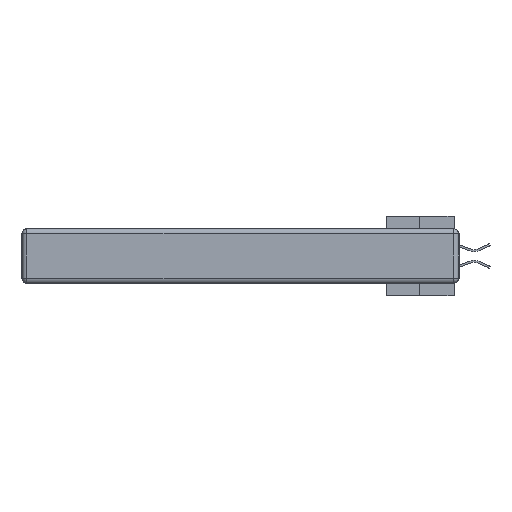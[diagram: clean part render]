
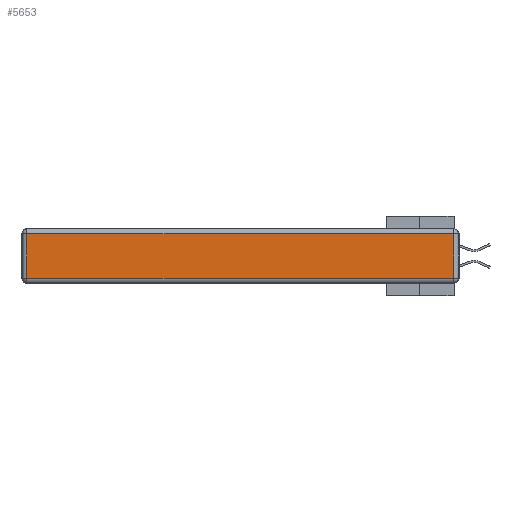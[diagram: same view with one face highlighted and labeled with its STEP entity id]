
A CAD part, left-side view. The second image highlights one B-rep face of the part: STEP entity #5653.
In plain terms, the highlighted planar face has unit normal (-1, 0, 0).
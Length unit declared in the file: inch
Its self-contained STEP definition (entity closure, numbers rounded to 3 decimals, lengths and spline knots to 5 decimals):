
#167 = VECTOR ( 'NONE', #23515, 39.37008 ) ;
#556 = VERTEX_POINT ( 'NONE', #31335 ) ;
#727 = EDGE_LOOP ( 'NONE', ( #11706, #19733, #2817, #20177 ) ) ;
#2817 = ORIENTED_EDGE ( 'NONE', *, *, #37532, .T. ) ;
#2846 = LINE ( 'NONE', #37188, #167 ) ;
#2944 = EDGE_CURVE ( 'NONE', #8887, #556, #6244, .T. ) ;
#5043 = VERTEX_POINT ( 'NONE', #32799 ) ;
#5653 = ADVANCED_FACE ( 'NONE', ( #38411 ), #18246, .T. ) ;
#5727 = CARTESIAN_POINT ( 'NONE',  ( 0., 0.03, -0.343 ) ) ;
#6244 = LINE ( 'NONE', #14846, #38567 ) ;
#8887 = VERTEX_POINT ( 'NONE', #13700 ) ;
#9393 = EDGE_CURVE ( 'NONE', #29796, #8887, #13921, .T. ) ;
#11181 = AXIS2_PLACEMENT_3D ( 'NONE', #21705, #21859, #15105 ) ;
#11333 = DIRECTION ( 'NONE',  ( 0., -1., 0. ) ) ;
#11706 = ORIENTED_EDGE ( 'NONE', *, *, #2944, .T. ) ;
#13700 = CARTESIAN_POINT ( 'NONE',  ( 0., 2.72, -0.313 ) ) ;
#13921 = LINE ( 'NONE', #23684, #37571 ) ;
#14846 = CARTESIAN_POINT ( 'NONE',  ( 0., 0., -0.313 ) ) ;
#15105 = DIRECTION ( 'NONE',  ( 0., 0., 1. ) ) ;
#18246 = PLANE ( 'NONE',  #11181 ) ;
#19733 = ORIENTED_EDGE ( 'NONE', *, *, #35099, .T. ) ;
#20177 = ORIENTED_EDGE ( 'NONE', *, *, #9393, .T. ) ;
#20609 = LINE ( 'NONE', #5727, #28678 ) ;
#21705 = CARTESIAN_POINT ( 'NONE',  ( 0., 0., -0.343 ) ) ;
#21859 = DIRECTION ( 'NONE',  ( -1., 0., 0. ) ) ;
#22917 = DIRECTION ( 'NONE',  ( 0., 0., 1. ) ) ;
#23515 = DIRECTION ( 'NONE',  ( 0., 1., 0. ) ) ;
#23684 = CARTESIAN_POINT ( 'NONE',  ( 0., 2.72, -0.343 ) ) ;
#28678 = VECTOR ( 'NONE', #22917, 39.37008 ) ;
#29796 = VERTEX_POINT ( 'NONE', #40499 ) ;
#31335 = CARTESIAN_POINT ( 'NONE',  ( 0., 0.03, -0.313 ) ) ;
#32799 = CARTESIAN_POINT ( 'NONE',  ( 0., 0.03, -0.03 ) ) ;
#33639 = DIRECTION ( 'NONE',  ( 0., 0., -1. ) ) ;
#35099 = EDGE_CURVE ( 'NONE', #556, #5043, #20609, .T. ) ;
#37188 = CARTESIAN_POINT ( 'NONE',  ( 0., 2.75, -0.03 ) ) ;
#37532 = EDGE_CURVE ( 'NONE', #5043, #29796, #2846, .T. ) ;
#37571 = VECTOR ( 'NONE', #33639, 39.37008 ) ;
#38411 = FACE_OUTER_BOUND ( 'NONE', #727, .T. ) ;
#38567 = VECTOR ( 'NONE', #11333, 39.37008 ) ;
#40499 = CARTESIAN_POINT ( 'NONE',  ( 0., 2.72, -0.03 ) ) ;
